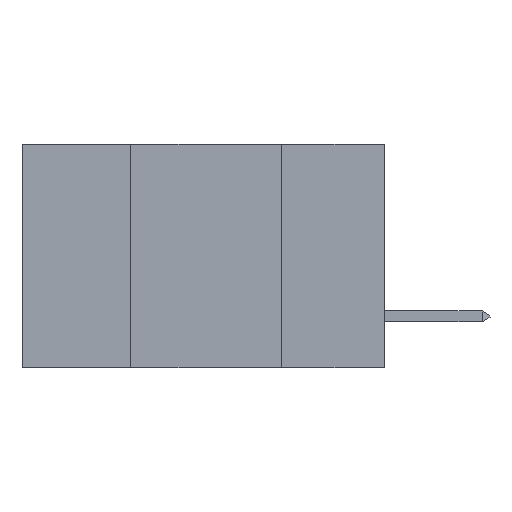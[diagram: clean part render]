
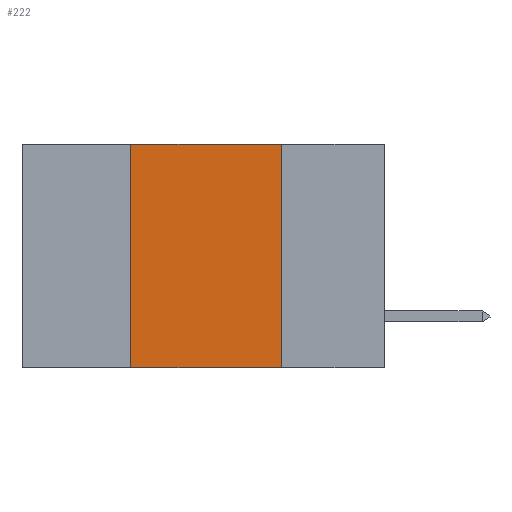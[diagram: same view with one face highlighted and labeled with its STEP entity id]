
A CAD part, left-side view. The second image highlights one B-rep face of the part: STEP entity #222.
In plain terms, the highlighted planar face has unit normal (-1, 0, 0).
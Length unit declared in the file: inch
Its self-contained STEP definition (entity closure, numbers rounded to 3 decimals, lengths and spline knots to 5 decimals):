
#93 = LINE ( 'NONE', #3528, #7022 ) ;
#222 = ADVANCED_FACE ( 'NONE', ( #12233 ), #3617, .F. ) ;
#331 = EDGE_CURVE ( 'NONE', #2999, #15308, #5766, .T. ) ;
#1270 = VERTEX_POINT ( 'NONE', #1794 ) ;
#1794 = CARTESIAN_POINT ( 'NONE',  ( 0., 0.17, -0.37 ) ) ;
#2040 = ORIENTED_EDGE ( 'NONE', *, *, #2761, .T. ) ;
#2232 = LINE ( 'NONE', #15012, #5392 ) ;
#2761 = EDGE_CURVE ( 'NONE', #14625, #1270, #7424, .T. ) ;
#2764 = EDGE_CURVE ( 'NONE', #14625, #2999, #93, .T. ) ;
#2849 = EDGE_CURVE ( 'NONE', #15308, #1270, #2232, .T. ) ;
#2973 = DIRECTION ( 'NONE',  ( 0., 0., 1. ) ) ;
#2999 = VERTEX_POINT ( 'NONE', #6846 ) ;
#3503 = CARTESIAN_POINT ( 'NONE',  ( 0., 0.6, -0.37 ) ) ;
#3528 = CARTESIAN_POINT ( 'NONE',  ( 0., 0.42, 0. ) ) ;
#3617 = PLANE ( 'NONE',  #8837 ) ;
#3884 = DIRECTION ( 'NONE',  ( 0., 0., -1. ) ) ;
#4418 = DIRECTION ( 'NONE',  ( 0., -1., 0. ) ) ;
#5392 = VECTOR ( 'NONE', #14794, 39.37008 ) ;
#5766 = LINE ( 'NONE', #11727, #15479 ) ;
#5999 = CARTESIAN_POINT ( 'NONE',  ( 0., 0.6, 0. ) ) ;
#6355 = ORIENTED_EDGE ( 'NONE', *, *, #2849, .F. ) ;
#6556 = ORIENTED_EDGE ( 'NONE', *, *, #331, .F. ) ;
#6576 = CARTESIAN_POINT ( 'NONE',  ( 0., 0.42, -0.37 ) ) ;
#6704 = DIRECTION ( 'NONE',  ( 1., 0., 0. ) ) ;
#6846 = CARTESIAN_POINT ( 'NONE',  ( 0., 0.42, 0. ) ) ;
#7022 = VECTOR ( 'NONE', #2973, 39.37008 ) ;
#7424 = LINE ( 'NONE', #3503, #13512 ) ;
#7532 = ORIENTED_EDGE ( 'NONE', *, *, #2764, .F. ) ;
#8837 = AXIS2_PLACEMENT_3D ( 'NONE', #5999, #6704, #3884 ) ;
#11626 = DIRECTION ( 'NONE',  ( 0., -1., 0. ) ) ;
#11727 = CARTESIAN_POINT ( 'NONE',  ( 0., 0.6, 0. ) ) ;
#12233 = FACE_OUTER_BOUND ( 'NONE', #12960, .T. ) ;
#12468 = CARTESIAN_POINT ( 'NONE',  ( 0., 0.17, 0. ) ) ;
#12960 = EDGE_LOOP ( 'NONE', ( #6355, #6556, #7532, #2040 ) ) ;
#13512 = VECTOR ( 'NONE', #4418, 39.37008 ) ;
#14625 = VERTEX_POINT ( 'NONE', #6576 ) ;
#14794 = DIRECTION ( 'NONE',  ( 0., 0., -1. ) ) ;
#15012 = CARTESIAN_POINT ( 'NONE',  ( 0., 0.17, 0. ) ) ;
#15308 = VERTEX_POINT ( 'NONE', #12468 ) ;
#15479 = VECTOR ( 'NONE', #11626, 39.37008 ) ;
